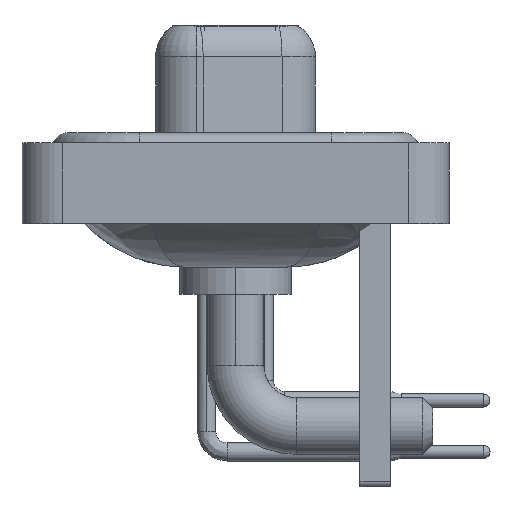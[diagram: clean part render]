
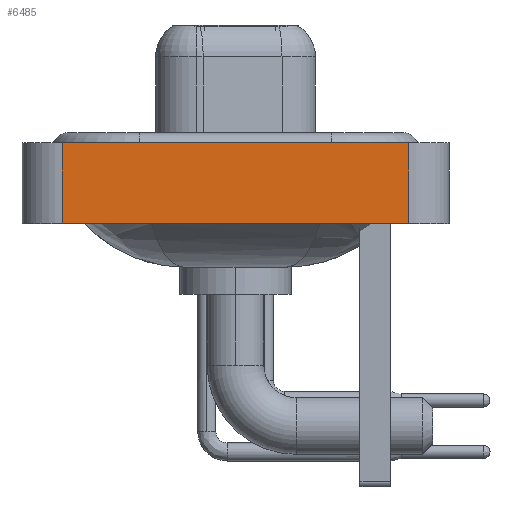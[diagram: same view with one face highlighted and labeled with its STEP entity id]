
A CAD part, left-side view. The second image highlights one B-rep face of the part: STEP entity #6485.
In plain terms, the highlighted planar face has unit normal (-1, 0, 0).
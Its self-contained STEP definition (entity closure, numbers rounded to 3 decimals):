
#880 = CARTESIAN_POINT ( 'NONE',  ( -7.35, 8.55, -3.6 ) ) ;
#1936 = EDGE_LOOP ( 'NONE', ( #14880, #18453, #12312, #17116 ) ) ;
#1966 = CARTESIAN_POINT ( 'NONE',  ( -7.35, -8.55, -3.6 ) ) ;
#2040 = VECTOR ( 'NONE', #9247, 1000. ) ;
#2276 = CARTESIAN_POINT ( 'NONE',  ( -7.35, -8.55, -3.6 ) ) ;
#2637 = VERTEX_POINT ( 'NONE', #2276 ) ;
#3224 = EDGE_CURVE ( 'NONE', #15005, #17858, #15850, .T. ) ;
#3606 = DIRECTION ( 'NONE',  ( 0., -1., 0. ) ) ;
#5152 = LINE ( 'NONE', #20447, #16089 ) ;
#5179 = PLANE ( 'NONE',  #14061 ) ;
#5381 = LINE ( 'NONE', #1966, #15014 ) ;
#6485 = ADVANCED_FACE ( 'NONE', ( #17040 ), #5179, .T. ) ;
#7776 = CARTESIAN_POINT ( 'NONE',  ( -7.35, 8.55, -3.6 ) ) ;
#8632 = CARTESIAN_POINT ( 'NONE',  ( -7.35, -8.55, -3.6 ) ) ;
#9244 = CARTESIAN_POINT ( 'NONE',  ( -7.35, 8.55, 0.4 ) ) ;
#9247 = DIRECTION ( 'NONE',  ( 0., 0., 1. ) ) ;
#10751 = DIRECTION ( 'NONE',  ( 0., 0., 1. ) ) ;
#12039 = DIRECTION ( 'NONE',  ( 0., 0., 1. ) ) ;
#12312 = ORIENTED_EDGE ( 'NONE', *, *, #3224, .F. ) ;
#14061 = AXIS2_PLACEMENT_3D ( 'NONE', #8632, #18915, #12039 ) ;
#14651 = LINE ( 'NONE', #21410, #2040 ) ;
#14880 = ORIENTED_EDGE ( 'NONE', *, *, #19283, .T. ) ;
#15005 = VERTEX_POINT ( 'NONE', #880 ) ;
#15014 = VECTOR ( 'NONE', #15681, 1000. ) ;
#15681 = DIRECTION ( 'NONE',  ( 0., -1., 0. ) ) ;
#15749 = EDGE_CURVE ( 'NONE', #15005, #2637, #5381, .T. ) ;
#15850 = LINE ( 'NONE', #7776, #17485 ) ;
#16089 = VECTOR ( 'NONE', #3606, 1000. ) ;
#17040 = FACE_OUTER_BOUND ( 'NONE', #1936, .T. ) ;
#17078 = CARTESIAN_POINT ( 'NONE',  ( -7.35, -8.55, 0.4 ) ) ;
#17116 = ORIENTED_EDGE ( 'NONE', *, *, #15749, .T. ) ;
#17485 = VECTOR ( 'NONE', #10751, 1000. ) ;
#17858 = VERTEX_POINT ( 'NONE', #9244 ) ;
#18453 = ORIENTED_EDGE ( 'NONE', *, *, #20952, .F. ) ;
#18915 = DIRECTION ( 'NONE',  ( -1., 0., 0. ) ) ;
#19283 = EDGE_CURVE ( 'NONE', #2637, #19942, #14651, .T. ) ;
#19942 = VERTEX_POINT ( 'NONE', #17078 ) ;
#20447 = CARTESIAN_POINT ( 'NONE',  ( -7.35, -8.55, 0.4 ) ) ;
#20952 = EDGE_CURVE ( 'NONE', #17858, #19942, #5152, .T. ) ;
#21410 = CARTESIAN_POINT ( 'NONE',  ( -7.35, -8.55, -3.6 ) ) ;
